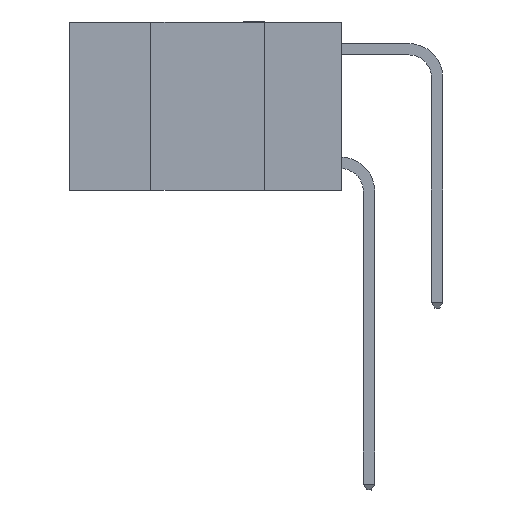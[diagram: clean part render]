
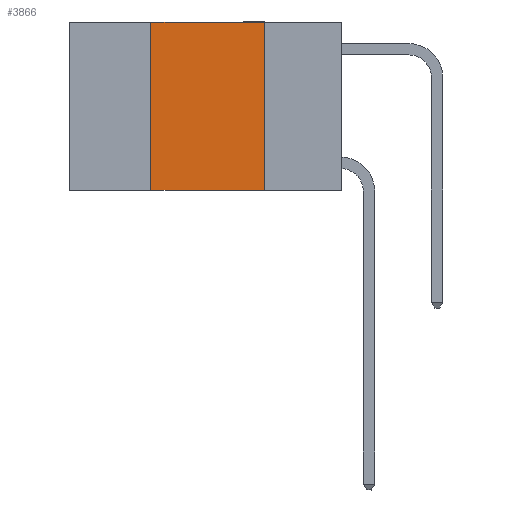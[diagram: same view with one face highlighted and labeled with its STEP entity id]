
A CAD part, left-side view. The second image highlights one B-rep face of the part: STEP entity #3866.
In plain terms, the highlighted planar face has unit normal (-1, 0, 0).
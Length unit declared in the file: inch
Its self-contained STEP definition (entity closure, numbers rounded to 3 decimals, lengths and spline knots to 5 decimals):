
#117 = DIRECTION ( 'NONE',  ( 0., 0., -1. ) ) ;
#625 = DIRECTION ( 'NONE',  ( 0., 0., -1. ) ) ;
#803 = LINE ( 'NONE', #4204, #11620 ) ;
#2239 = EDGE_CURVE ( 'NONE', #13474, #6123, #3785, .T. ) ;
#2515 = EDGE_CURVE ( 'NONE', #13474, #5954, #803, .T. ) ;
#3145 = VERTEX_POINT ( 'NONE', #8939 ) ;
#3785 = LINE ( 'NONE', #6669, #11314 ) ;
#3866 = ADVANCED_FACE ( 'NONE', ( #4474 ), #12638, .F. ) ;
#4204 = CARTESIAN_POINT ( 'NONE',  ( 0., 0.6, -0.37 ) ) ;
#4474 = FACE_OUTER_BOUND ( 'NONE', #12183, .T. ) ;
#5239 = DIRECTION ( 'NONE',  ( 0., -1., 0. ) ) ;
#5557 = LINE ( 'NONE', #12209, #10511 ) ;
#5954 = VERTEX_POINT ( 'NONE', #12066 ) ;
#6123 = VERTEX_POINT ( 'NONE', #8237 ) ;
#6171 = CARTESIAN_POINT ( 'NONE',  ( 0., 0.42, -0.37 ) ) ;
#6666 = DIRECTION ( 'NONE',  ( 1., 0., 0. ) ) ;
#6669 = CARTESIAN_POINT ( 'NONE',  ( 0., 0.42, 0. ) ) ;
#6917 = DIRECTION ( 'NONE',  ( 0., -1., 0. ) ) ;
#7245 = ORIENTED_EDGE ( 'NONE', *, *, #2515, .T. ) ;
#8190 = ORIENTED_EDGE ( 'NONE', *, *, #2239, .F. ) ;
#8226 = DIRECTION ( 'NONE',  ( 0., 0., 1. ) ) ;
#8237 = CARTESIAN_POINT ( 'NONE',  ( 0., 0.42, 0. ) ) ;
#8841 = AXIS2_PLACEMENT_3D ( 'NONE', #10599, #6666, #117 ) ;
#8939 = CARTESIAN_POINT ( 'NONE',  ( 0., 0.17, 0. ) ) ;
#8979 = EDGE_CURVE ( 'NONE', #6123, #3145, #5557, .T. ) ;
#9231 = VECTOR ( 'NONE', #625, 39.37008 ) ;
#9400 = ORIENTED_EDGE ( 'NONE', *, *, #8979, .F. ) ;
#9885 = EDGE_CURVE ( 'NONE', #3145, #5954, #11914, .T. ) ;
#10511 = VECTOR ( 'NONE', #5239, 39.37008 ) ;
#10599 = CARTESIAN_POINT ( 'NONE',  ( 0., 0.6, 0. ) ) ;
#11314 = VECTOR ( 'NONE', #8226, 39.37008 ) ;
#11620 = VECTOR ( 'NONE', #6917, 39.37008 ) ;
#11914 = LINE ( 'NONE', #12104, #9231 ) ;
#12066 = CARTESIAN_POINT ( 'NONE',  ( 0., 0.17, -0.37 ) ) ;
#12085 = ORIENTED_EDGE ( 'NONE', *, *, #9885, .F. ) ;
#12104 = CARTESIAN_POINT ( 'NONE',  ( 0., 0.17, 0. ) ) ;
#12183 = EDGE_LOOP ( 'NONE', ( #12085, #9400, #8190, #7245 ) ) ;
#12209 = CARTESIAN_POINT ( 'NONE',  ( 0., 0.6, 0. ) ) ;
#12638 = PLANE ( 'NONE',  #8841 ) ;
#13474 = VERTEX_POINT ( 'NONE', #6171 ) ;
